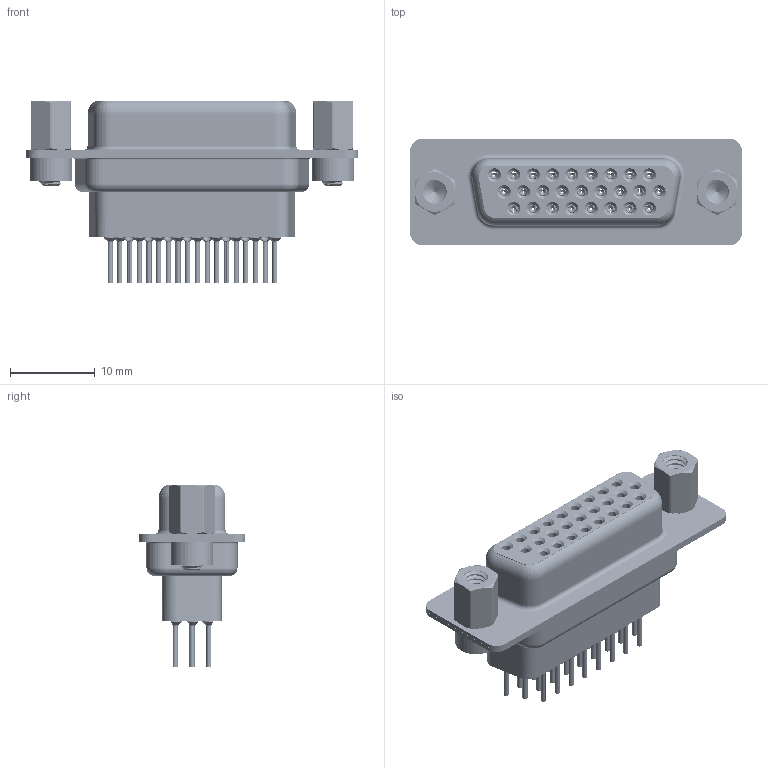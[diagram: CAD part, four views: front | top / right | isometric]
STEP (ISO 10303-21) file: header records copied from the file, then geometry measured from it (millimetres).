
FILE_DESCRIPTION (( 'STEP AP203' ), '1' );
FILE_NAME ('638-026-331-073.STEP', '2020-07-18T20:40:38', ( '' ), ( '' ), 'SwSTEP 2.0', 'SolidWorks 2020', '' );
FILE_SCHEMA (( 'CONFIG_CONTROL_DESIGN' ));
Length unit declared in the file: millimetre
Products named in the file (9): 638 Contact Row 1_31; 638 Contact Row 3_31; 638 Shell Front_26 Contacts; 638 4-40 Hex Standoff; 638 Shell Rear_26 Contacts; 638 4-40 Threaded Rivet; 638-026-331-073; 638 Housing_26 Contacts HP; 638 Contact Row 2_31
Assembly tree (33 placements, depth 2):
  638-026-331-073
    638 Housing_26 Contacts HP
    638 Shell Front_26 Contacts
    638 Shell Rear_26 Contacts
    638 Contact Row 1_31  x9
    638 Contact Row 2_31  x9
    638 Contact Row 3_31  x8
    638 4-40 Threaded Rivet  x2
    638 4-40 Hex Standoff  x2
Bounding box: 39.19 x 12.6 x 21.5 mm (x, y, z)
Volume: 2889.4 mm3; surface area: 10355.3 mm2
Topology: 33 solids, 33 shells, 3603 faces, 9249 edges, 5775 vertices
Faces by surface type: cylinder 1067, plane 895, torus 681, bspline 538, cone 422
Entity records: 37372 total; most frequent: CARTESIAN_POINT 12964, DIRECTION 4883, ORIENTED_EDGE 4730, EDGE_CURVE 2365, AXIS2_PLACEMENT_3D 2033, VERTEX_POINT 1493, EDGE_LOOP 1132, CIRCLE 1089
